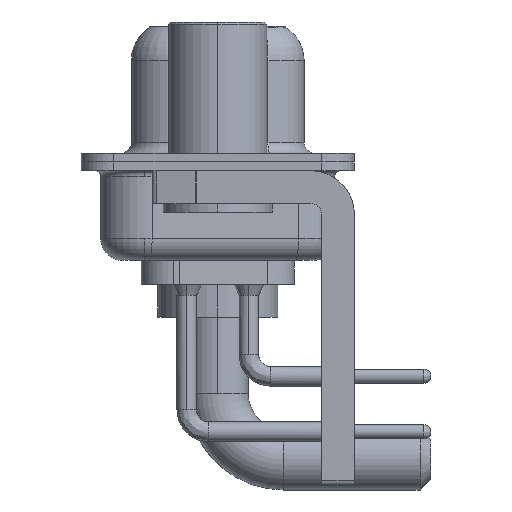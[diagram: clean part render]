
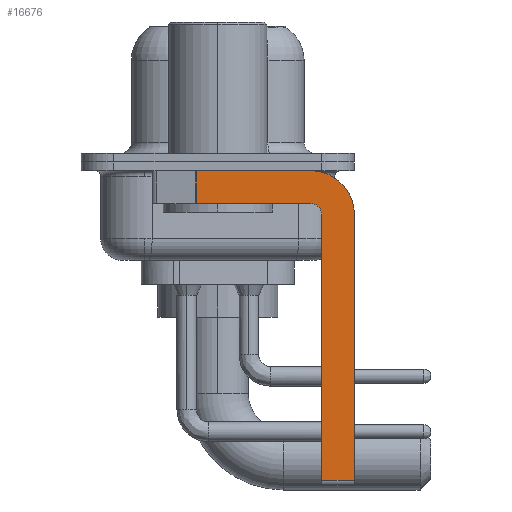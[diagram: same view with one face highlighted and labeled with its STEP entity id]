
A CAD part, left-side view. The second image highlights one B-rep face of the part: STEP entity #16676.
In plain terms, the highlighted planar face has unit normal (-1, 0, 0).
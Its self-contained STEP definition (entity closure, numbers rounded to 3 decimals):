
#15 = EDGE_CURVE ( 'NONE', #1953, #6595, #1926, .T. ) ;
#299 = DIRECTION ( 'NONE',  ( 1., 0., 0. ) ) ;
#530 = CARTESIAN_POINT ( 'NONE',  ( -2.9, -4.25, -0.4 ) ) ;
#830 = AXIS2_PLACEMENT_3D ( 'NONE', #10428, #299, #4397 ) ;
#1192 = CARTESIAN_POINT ( 'NONE',  ( -2.9, -4.25, -2.4 ) ) ;
#1540 = VECTOR ( 'NONE', #16429, 1000. ) ;
#1926 = LINE ( 'NONE', #3638, #17842 ) ;
#1953 = VERTEX_POINT ( 'NONE', #11751 ) ;
#2267 = VECTOR ( 'NONE', #4592, 1000. ) ;
#2286 = LINE ( 'NONE', #15434, #14139 ) ;
#2477 = ORIENTED_EDGE ( 'NONE', *, *, #14943, .T. ) ;
#2881 = LINE ( 'NONE', #8713, #6931 ) ;
#2949 = AXIS2_PLACEMENT_3D ( 'NONE', #1192, #12661, #14027 ) ;
#3564 = CIRCLE ( 'NONE', #2949, 0.5 ) ;
#3638 = CARTESIAN_POINT ( 'NONE',  ( -2.9, -4.75, -14.8 ) ) ;
#3881 = ORIENTED_EDGE ( 'NONE', *, *, #18644, .F. ) ;
#4262 = CARTESIAN_POINT ( 'NONE',  ( -2.9, 0.978, -0.4 ) ) ;
#4397 = DIRECTION ( 'NONE',  ( 0., 0., -1. ) ) ;
#4592 = DIRECTION ( 'NONE',  ( 0., -1., 0. ) ) ;
#4687 = CARTESIAN_POINT ( 'NONE',  ( -2.9, -4.25, -14.55 ) ) ;
#5168 = VERTEX_POINT ( 'NONE', #15801 ) ;
#5652 = AXIS2_PLACEMENT_3D ( 'NONE', #9938, #15652, #5726 ) ;
#5687 = CARTESIAN_POINT ( 'NONE',  ( -2.9, 0.978, -1.9 ) ) ;
#5726 = DIRECTION ( 'NONE',  ( 0., 0., -1. ) ) ;
#5899 = EDGE_CURVE ( 'NONE', #14352, #12732, #15276, .T. ) ;
#6035 = LINE ( 'NONE', #4687, #2267 ) ;
#6595 = VERTEX_POINT ( 'NONE', #10920 ) ;
#6797 = DIRECTION ( 'NONE',  ( 0., 1., 0. ) ) ;
#6931 = VECTOR ( 'NONE', #6797, 1000. ) ;
#7189 = VERTEX_POINT ( 'NONE', #17923 ) ;
#7424 = VECTOR ( 'NONE', #17749, 1000. ) ;
#7741 = CARTESIAN_POINT ( 'NONE',  ( -2.9, 0.978, -1.9 ) ) ;
#8201 = DIRECTION ( 'NONE',  ( 0., 0., -1. ) ) ;
#8713 = CARTESIAN_POINT ( 'NONE',  ( -2.9, -4.25, -1.9 ) ) ;
#8905 = CARTESIAN_POINT ( 'NONE',  ( -2.9, 3., -0.4 ) ) ;
#9257 = ORIENTED_EDGE ( 'NONE', *, *, #14333, .F. ) ;
#9342 = EDGE_LOOP ( 'NONE', ( #17940, #16587, #3881, #11790, #18687, #2477, #9257, #12040 ) ) ;
#9479 = DIRECTION ( 'NONE',  ( 0., 0., 1. ) ) ;
#9938 = CARTESIAN_POINT ( 'NONE',  ( -2.9, -4.25, -2.4 ) ) ;
#10428 = CARTESIAN_POINT ( 'NONE',  ( -2.9, -4.25, -2.4 ) ) ;
#10628 = LINE ( 'NONE', #8905, #7424 ) ;
#10734 = VERTEX_POINT ( 'NONE', #18662 ) ;
#10920 = CARTESIAN_POINT ( 'NONE',  ( -2.9, -4.75, -2.4 ) ) ;
#11563 = PLANE ( 'NONE',  #5652 ) ;
#11751 = CARTESIAN_POINT ( 'NONE',  ( -2.9, -4.75, -14.55 ) ) ;
#11790 = ORIENTED_EDGE ( 'NONE', *, *, #17603, .F. ) ;
#12040 = ORIENTED_EDGE ( 'NONE', *, *, #18694, .F. ) ;
#12661 = DIRECTION ( 'NONE',  ( -1., 0., 0. ) ) ;
#12732 = VERTEX_POINT ( 'NONE', #5687 ) ;
#12881 = VERTEX_POINT ( 'NONE', #530 ) ;
#13637 = CIRCLE ( 'NONE', #830, 2. ) ;
#14027 = DIRECTION ( 'NONE',  ( 0., 0., 1. ) ) ;
#14139 = VECTOR ( 'NONE', #8201, 1000. ) ;
#14333 = EDGE_CURVE ( 'NONE', #10734, #5168, #2286, .T. ) ;
#14352 = VERTEX_POINT ( 'NONE', #4262 ) ;
#14936 = EDGE_CURVE ( 'NONE', #14352, #12881, #10628, .T. ) ;
#14943 = EDGE_CURVE ( 'NONE', #1953, #5168, #6035, .T. ) ;
#15276 = LINE ( 'NONE', #7741, #1540 ) ;
#15304 = FACE_OUTER_BOUND ( 'NONE', #9342, .T. ) ;
#15434 = CARTESIAN_POINT ( 'NONE',  ( -2.9, -6.25, -2.4 ) ) ;
#15652 = DIRECTION ( 'NONE',  ( 1., 0., 0. ) ) ;
#15801 = CARTESIAN_POINT ( 'NONE',  ( -2.9, -6.25, -14.55 ) ) ;
#16429 = DIRECTION ( 'NONE',  ( 0., 0., -1. ) ) ;
#16587 = ORIENTED_EDGE ( 'NONE', *, *, #5899, .T. ) ;
#16676 = ADVANCED_FACE ( 'NONE', ( #15304 ), #11563, .F. ) ;
#17603 = EDGE_CURVE ( 'NONE', #6595, #7189, #3564, .T. ) ;
#17749 = DIRECTION ( 'NONE',  ( 0., -1., 0. ) ) ;
#17842 = VECTOR ( 'NONE', #9479, 1000. ) ;
#17923 = CARTESIAN_POINT ( 'NONE',  ( -2.9, -4.25, -1.9 ) ) ;
#17940 = ORIENTED_EDGE ( 'NONE', *, *, #14936, .F. ) ;
#18644 = EDGE_CURVE ( 'NONE', #7189, #12732, #2881, .T. ) ;
#18662 = CARTESIAN_POINT ( 'NONE',  ( -2.9, -6.25, -2.4 ) ) ;
#18687 = ORIENTED_EDGE ( 'NONE', *, *, #15, .F. ) ;
#18694 = EDGE_CURVE ( 'NONE', #12881, #10734, #13637, .T. ) ;
